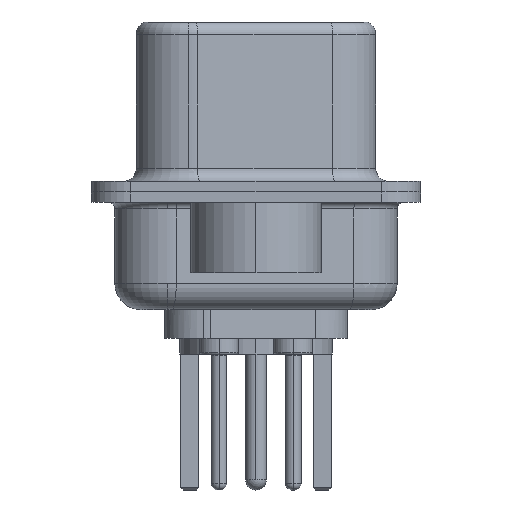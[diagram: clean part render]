
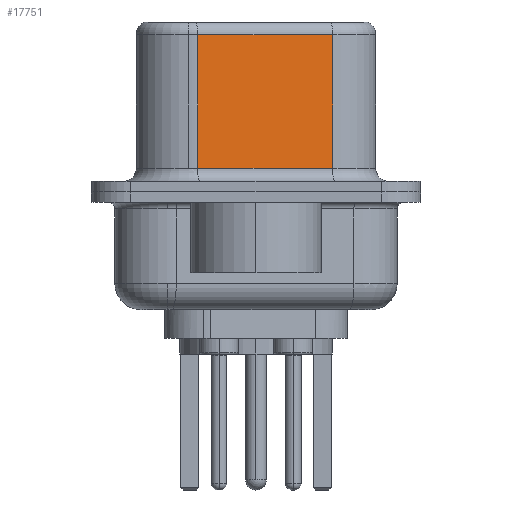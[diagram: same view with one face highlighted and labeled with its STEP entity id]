
A CAD part, left-side view. The second image highlights one B-rep face of the part: STEP entity #17751.
In plain terms, the highlighted planar face has unit normal (-0.985, -0.174, 0).
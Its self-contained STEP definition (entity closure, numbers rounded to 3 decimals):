
#207 = CARTESIAN_POINT ( 'NONE',  ( 4.565, -2.927, 6.02 ) ) ;
#318 = CARTESIAN_POINT ( 'NONE',  ( 3.655, 2.233, 6.52 ) ) ;
#398 = LINE ( 'NONE', #318, #17867 ) ;
#941 = ORIENTED_EDGE ( 'NONE', *, *, #12455, .F. ) ;
#2126 = EDGE_CURVE ( 'NONE', #20269, #7058, #398, .T. ) ;
#2269 = DIRECTION ( 'NONE',  ( 0.174, -0.985, 0. ) ) ;
#2301 = DIRECTION ( 'NONE',  ( 0., 0., -1. ) ) ;
#2547 = CARTESIAN_POINT ( 'NONE',  ( 4.565, -2.927, 6.52 ) ) ;
#3871 = VECTOR ( 'NONE', #12628, 1000. ) ;
#4276 = VERTEX_POINT ( 'NONE', #6814 ) ;
#4288 = DIRECTION ( 'NONE',  ( -0.174, 0.985, 0. ) ) ;
#4510 = VECTOR ( 'NONE', #15687, 1000. ) ;
#5593 = LINE ( 'NONE', #207, #4510 ) ;
#6814 = CARTESIAN_POINT ( 'NONE',  ( 4.565, -2.927, 0.9 ) ) ;
#7058 = VERTEX_POINT ( 'NONE', #20634 ) ;
#8238 = VECTOR ( 'NONE', #2269, 1000. ) ;
#8723 = EDGE_CURVE ( 'NONE', #19289, #20269, #5593, .T. ) ;
#9524 = ORIENTED_EDGE ( 'NONE', *, *, #2126, .T. ) ;
#10954 = CARTESIAN_POINT ( 'NONE',  ( 3.655, 2.233, 6.02 ) ) ;
#11240 = EDGE_CURVE ( 'NONE', #7058, #4276, #13526, .T. ) ;
#11811 = AXIS2_PLACEMENT_3D ( 'NONE', #2547, #14779, #4288 ) ;
#12455 = EDGE_CURVE ( 'NONE', #19289, #4276, #16799, .T. ) ;
#12628 = DIRECTION ( 'NONE',  ( 0., 0., -1. ) ) ;
#12766 = CARTESIAN_POINT ( 'NONE',  ( 4.565, -2.927, 0.9 ) ) ;
#13057 = PLANE ( 'NONE',  #11811 ) ;
#13526 = LINE ( 'NONE', #12766, #8238 ) ;
#14779 = DIRECTION ( 'NONE',  ( 0.985, 0.174, 0. ) ) ;
#15385 = ORIENTED_EDGE ( 'NONE', *, *, #8723, .T. ) ;
#15556 = CARTESIAN_POINT ( 'NONE',  ( 4.565, -2.927, 6.02 ) ) ;
#15671 = FACE_OUTER_BOUND ( 'NONE', #17002, .T. ) ;
#15687 = DIRECTION ( 'NONE',  ( -0.174, 0.985, 0. ) ) ;
#16799 = LINE ( 'NONE', #18041, #3871 ) ;
#17002 = EDGE_LOOP ( 'NONE', ( #941, #15385, #9524, #21517 ) ) ;
#17751 = ADVANCED_FACE ( 'NONE', ( #15671 ), #13057, .F. ) ;
#17867 = VECTOR ( 'NONE', #2301, 1000. ) ;
#18041 = CARTESIAN_POINT ( 'NONE',  ( 4.565, -2.927, 6.52 ) ) ;
#19289 = VERTEX_POINT ( 'NONE', #15556 ) ;
#20269 = VERTEX_POINT ( 'NONE', #10954 ) ;
#20634 = CARTESIAN_POINT ( 'NONE',  ( 3.655, 2.233, 0.9 ) ) ;
#21517 = ORIENTED_EDGE ( 'NONE', *, *, #11240, .T. ) ;
